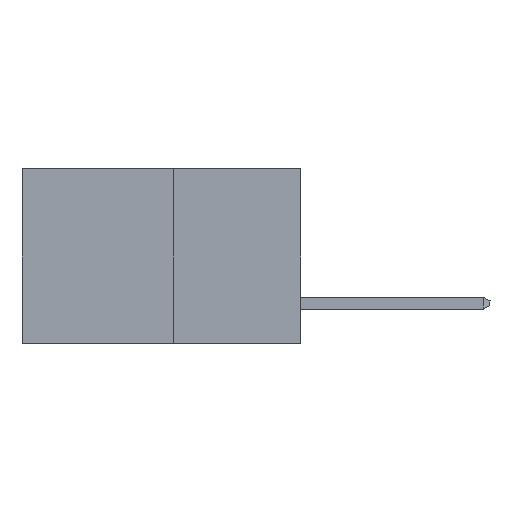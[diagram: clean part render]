
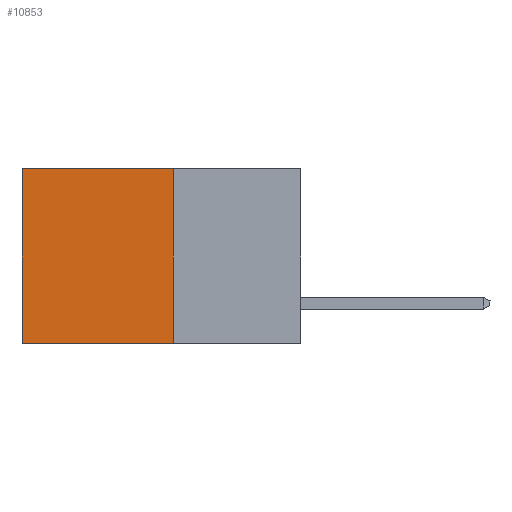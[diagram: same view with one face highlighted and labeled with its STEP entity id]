
A CAD part, left-side view. The second image highlights one B-rep face of the part: STEP entity #10853.
In plain terms, the highlighted planar face has unit normal (-1, 0, 0).
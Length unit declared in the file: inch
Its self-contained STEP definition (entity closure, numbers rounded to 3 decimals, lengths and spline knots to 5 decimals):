
#189 = CARTESIAN_POINT ( 'NONE',  ( 0.277, 0.27, -0.37 ) ) ;
#294 = LINE ( 'NONE', #189, #15990 ) ;
#430 = VERTEX_POINT ( 'NONE', #10316 ) ;
#1679 = CARTESIAN_POINT ( 'NONE',  ( 0.277, 0.27, -0.37 ) ) ;
#2273 = LINE ( 'NONE', #1679, #15394 ) ;
#2482 = DIRECTION ( 'NONE',  ( 0., 0., -1. ) ) ;
#2819 = ORIENTED_EDGE ( 'NONE', *, *, #11605, .T. ) ;
#2992 = CARTESIAN_POINT ( 'NONE',  ( 0.277, 0.59, -0.37 ) ) ;
#3228 = EDGE_CURVE ( 'NONE', #430, #12681, #12767, .T. ) ;
#3369 = VERTEX_POINT ( 'NONE', #9786 ) ;
#4299 = DIRECTION ( 'NONE',  ( 0., 0., -1. ) ) ;
#5087 = FACE_OUTER_BOUND ( 'NONE', #6493, .T. ) ;
#6493 = EDGE_LOOP ( 'NONE', ( #2819, #7405, #7501, #7557 ) ) ;
#7405 = ORIENTED_EDGE ( 'NONE', *, *, #13357, .F. ) ;
#7501 = ORIENTED_EDGE ( 'NONE', *, *, #14424, .F. ) ;
#7557 = ORIENTED_EDGE ( 'NONE', *, *, #3228, .T. ) ;
#7900 = VECTOR ( 'NONE', #10714, 39.37008 ) ;
#8204 = VERTEX_POINT ( 'NONE', #9986 ) ;
#9428 = VECTOR ( 'NONE', #12863, 39.37008 ) ;
#9786 = CARTESIAN_POINT ( 'NONE',  ( 0.277, 0.27, -0.37 ) ) ;
#9986 = CARTESIAN_POINT ( 'NONE',  ( 0.277, 0.59, -0.37 ) ) ;
#10201 = DIRECTION ( 'NONE',  ( 1., 0., 0. ) ) ;
#10316 = CARTESIAN_POINT ( 'NONE',  ( 0.277, 0.27, 0. ) ) ;
#10500 = DIRECTION ( 'NONE',  ( 0., 1., 0. ) ) ;
#10714 = DIRECTION ( 'NONE',  ( 0., 0., -1. ) ) ;
#10853 = ADVANCED_FACE ( 'NONE', ( #5087 ), #16347, .F. ) ;
#11605 = EDGE_CURVE ( 'NONE', #12681, #8204, #14201, .T. ) ;
#12681 = VERTEX_POINT ( 'NONE', #12952 ) ;
#12767 = LINE ( 'NONE', #12931, #9428 ) ;
#12863 = DIRECTION ( 'NONE',  ( 0., 1., 0. ) ) ;
#12931 = CARTESIAN_POINT ( 'NONE',  ( 0.277, 0.27, 0. ) ) ;
#12952 = CARTESIAN_POINT ( 'NONE',  ( 0.277, 0.59, 0. ) ) ;
#13357 = EDGE_CURVE ( 'NONE', #3369, #8204, #294, .T. ) ;
#13960 = CARTESIAN_POINT ( 'NONE',  ( 0.277, 0.27, -0.37 ) ) ;
#14201 = LINE ( 'NONE', #2992, #7900 ) ;
#14282 = AXIS2_PLACEMENT_3D ( 'NONE', #13960, #10201, #2482 ) ;
#14424 = EDGE_CURVE ( 'NONE', #430, #3369, #2273, .T. ) ;
#15394 = VECTOR ( 'NONE', #4299, 39.37008 ) ;
#15990 = VECTOR ( 'NONE', #10500, 39.37008 ) ;
#16347 = PLANE ( 'NONE',  #14282 ) ;
